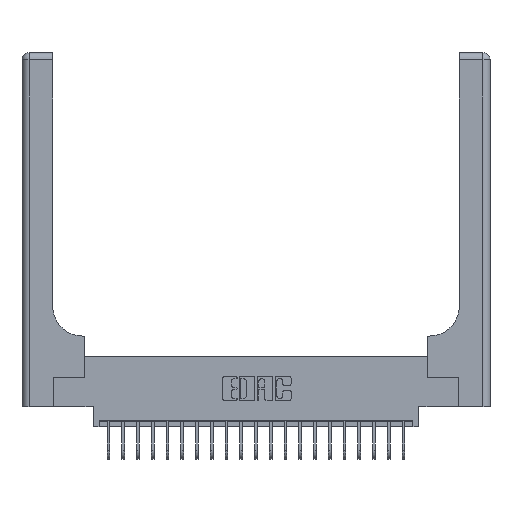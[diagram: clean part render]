
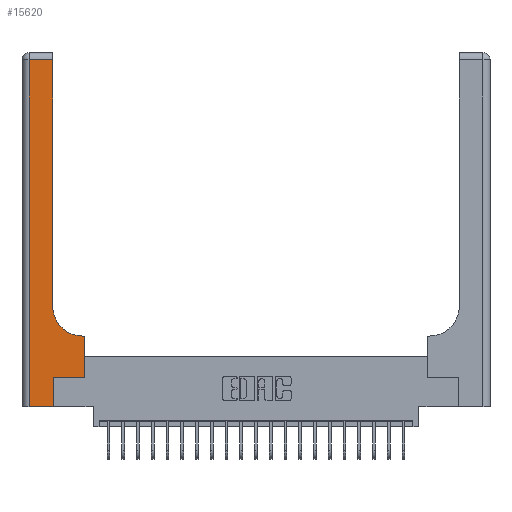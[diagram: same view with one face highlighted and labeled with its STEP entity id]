
A CAD part, top view. The second image highlights one B-rep face of the part: STEP entity #15620.
In plain terms, the highlighted planar face has unit normal (0, 0, 1).
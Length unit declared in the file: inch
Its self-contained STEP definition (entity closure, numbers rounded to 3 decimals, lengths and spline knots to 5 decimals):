
#215 = VECTOR ( 'NONE', #4364, 39.37008 ) ;
#329 = CARTESIAN_POINT ( 'NONE',  ( 0.265, 0.25, 0.37 ) ) ;
#398 = CARTESIAN_POINT ( 'NONE',  ( 0.26, 0.85, 0.37 ) ) ;
#524 = CARTESIAN_POINT ( 'NONE',  ( 0.51, 0.85, 0.37 ) ) ;
#662 = VERTEX_POINT ( 'NONE', #12508 ) ;
#720 = EDGE_LOOP ( 'NONE', ( #10297, #13074, #7521, #10374, #15737, #5051, #17118, #16337, #14646 ) ) ;
#999 = CARTESIAN_POINT ( 'NONE',  ( 0., 3., 0.37 ) ) ;
#1198 = FACE_OUTER_BOUND ( 'NONE', #720, .T. ) ;
#1227 = CARTESIAN_POINT ( 'NONE',  ( 0.26, 0.6, 0.37 ) ) ;
#1576 = CARTESIAN_POINT ( 'NONE',  ( 0.06, 0., 0.37 ) ) ;
#1880 = CARTESIAN_POINT ( 'NONE',  ( 0.26, 2.94, 0.37 ) ) ;
#1983 = EDGE_CURVE ( 'NONE', #15811, #16944, #4663, .T. ) ;
#2024 = DIRECTION ( 'NONE',  ( 1., 0., 0. ) ) ;
#2040 = DIRECTION ( 'NONE',  ( 0., 1., 0. ) ) ;
#2214 = DIRECTION ( 'NONE',  ( 1., 0., 0. ) ) ;
#2681 = PLANE ( 'NONE',  #15382 ) ;
#2897 = DIRECTION ( 'NONE',  ( -1., 0., 0. ) ) ;
#3086 = AXIS2_PLACEMENT_3D ( 'NONE', #524, #12053, #2214 ) ;
#4340 = DIRECTION ( 'NONE',  ( -1., 0., 0. ) ) ;
#4347 = LINE ( 'NONE', #20233, #4867 ) ;
#4364 = DIRECTION ( 'NONE',  ( 0., 1., 0. ) ) ;
#4499 = EDGE_CURVE ( 'NONE', #662, #19851, #12772, .T. ) ;
#4599 = EDGE_CURVE ( 'NONE', #11177, #10100, #12270, .T. ) ;
#4663 = LINE ( 'NONE', #15844, #215 ) ;
#4867 = VECTOR ( 'NONE', #8865, 39.37008 ) ;
#5051 = ORIENTED_EDGE ( 'NONE', *, *, #11133, .T. ) ;
#5069 = EDGE_CURVE ( 'NONE', #9597, #11177, #6386, .T. ) ;
#5087 = CARTESIAN_POINT ( 'NONE',  ( 0.265, 0.25, 0.37 ) ) ;
#5710 = VECTOR ( 'NONE', #10745, 39.37008 ) ;
#6228 = LINE ( 'NONE', #18901, #5710 ) ;
#6290 = VECTOR ( 'NONE', #2024, 39.37008 ) ;
#6386 = CIRCLE ( 'NONE', #3086, 0.25 ) ;
#6814 = LINE ( 'NONE', #329, #6290 ) ;
#6933 = VECTOR ( 'NONE', #15821, 39.37008 ) ;
#7082 = CARTESIAN_POINT ( 'NONE',  ( 0.51, 0.6, 0.37 ) ) ;
#7382 = VECTOR ( 'NONE', #2897, 39.37008 ) ;
#7521 = ORIENTED_EDGE ( 'NONE', *, *, #4499, .T. ) ;
#8471 = VECTOR ( 'NONE', #12292, 39.37008 ) ;
#8865 = DIRECTION ( 'NONE',  ( 1., 0., 0. ) ) ;
#9597 = VERTEX_POINT ( 'NONE', #7082 ) ;
#10100 = VERTEX_POINT ( 'NONE', #1880 ) ;
#10297 = ORIENTED_EDGE ( 'NONE', *, *, #4599, .T. ) ;
#10374 = ORIENTED_EDGE ( 'NONE', *, *, #14923, .T. ) ;
#10745 = DIRECTION ( 'NONE',  ( -1., 0., 0. ) ) ;
#11133 = EDGE_CURVE ( 'NONE', #19294, #15811, #6814, .T. ) ;
#11177 = VERTEX_POINT ( 'NONE', #398 ) ;
#11983 = LINE ( 'NONE', #15186, #20162 ) ;
#12053 = DIRECTION ( 'NONE',  ( 0., 0., -1. ) ) ;
#12270 = LINE ( 'NONE', #17392, #6933 ) ;
#12292 = DIRECTION ( 'NONE',  ( 0., -1., 0. ) ) ;
#12508 = CARTESIAN_POINT ( 'NONE',  ( 0.06, 2.94, 0.37 ) ) ;
#12772 = LINE ( 'NONE', #20423, #8471 ) ;
#13074 = ORIENTED_EDGE ( 'NONE', *, *, #13812, .T. ) ;
#13812 = EDGE_CURVE ( 'NONE', #10100, #662, #6228, .T. ) ;
#14087 = DIRECTION ( 'NONE',  ( 0., 0., -1. ) ) ;
#14646 = ORIENTED_EDGE ( 'NONE', *, *, #5069, .T. ) ;
#14923 = EDGE_CURVE ( 'NONE', #19851, #20344, #4347, .T. ) ;
#15186 = CARTESIAN_POINT ( 'NONE',  ( 0.265, 0., 0.37 ) ) ;
#15382 = AXIS2_PLACEMENT_3D ( 'NONE', #999, #14087, #4340 ) ;
#15620 = ADVANCED_FACE ( 'NONE', ( #1198 ), #2681, .F. ) ;
#15737 = ORIENTED_EDGE ( 'NONE', *, *, #21126, .T. ) ;
#15811 = VERTEX_POINT ( 'NONE', #16254 ) ;
#15821 = DIRECTION ( 'NONE',  ( 0., 1., 0. ) ) ;
#15844 = CARTESIAN_POINT ( 'NONE',  ( 0.528, 0.25, 0.37 ) ) ;
#16050 = LINE ( 'NONE', #1227, #7382 ) ;
#16254 = CARTESIAN_POINT ( 'NONE',  ( 0.528, 0.25, 0.37 ) ) ;
#16337 = ORIENTED_EDGE ( 'NONE', *, *, #18344, .T. ) ;
#16944 = VERTEX_POINT ( 'NONE', #20342 ) ;
#17118 = ORIENTED_EDGE ( 'NONE', *, *, #1983, .T. ) ;
#17392 = CARTESIAN_POINT ( 'NONE',  ( 0.26, 3., 0.37 ) ) ;
#18344 = EDGE_CURVE ( 'NONE', #16944, #9597, #16050, .T. ) ;
#18845 = CARTESIAN_POINT ( 'NONE',  ( 0.265, 0., 0.37 ) ) ;
#18901 = CARTESIAN_POINT ( 'NONE',  ( 0., 2.94, 0.37 ) ) ;
#19294 = VERTEX_POINT ( 'NONE', #5087 ) ;
#19851 = VERTEX_POINT ( 'NONE', #1576 ) ;
#20162 = VECTOR ( 'NONE', #2040, 39.37008 ) ;
#20233 = CARTESIAN_POINT ( 'NONE',  ( 0., 0., 0.37 ) ) ;
#20342 = CARTESIAN_POINT ( 'NONE',  ( 0.528, 0.6, 0.37 ) ) ;
#20344 = VERTEX_POINT ( 'NONE', #18845 ) ;
#20423 = CARTESIAN_POINT ( 'NONE',  ( 0.06, 3., 0.37 ) ) ;
#21126 = EDGE_CURVE ( 'NONE', #20344, #19294, #11983, .T. ) ;
